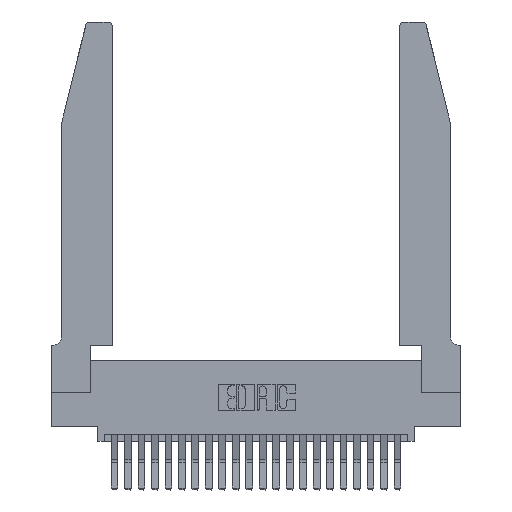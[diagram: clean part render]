
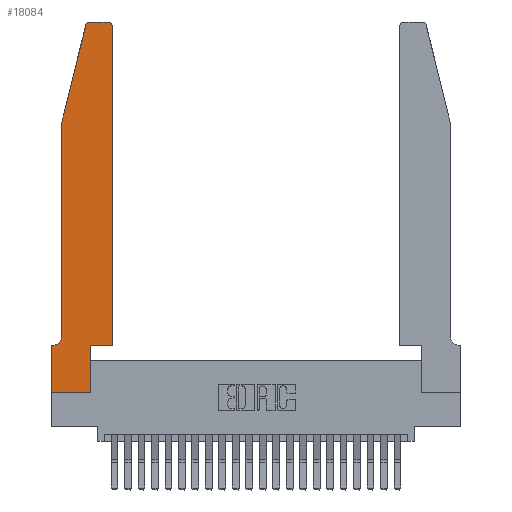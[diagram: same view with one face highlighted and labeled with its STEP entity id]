
A CAD part, top view. The second image highlights one B-rep face of the part: STEP entity #18084.
In plain terms, the highlighted planar face has unit normal (0, 0, 1).
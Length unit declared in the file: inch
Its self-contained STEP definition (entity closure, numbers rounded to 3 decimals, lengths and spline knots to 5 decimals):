
#71 = LINE ( 'NONE', #7031, #2191 ) ;
#272 = LINE ( 'NONE', #7744, #11992 ) ;
#812 = LINE ( 'NONE', #16373, #2931 ) ;
#839 = CARTESIAN_POINT ( 'NONE',  ( 0.0755, 0.42, 0.37 ) ) ;
#1042 = VERTEX_POINT ( 'NONE', #2028 ) ;
#1114 = EDGE_CURVE ( 'NONE', #1042, #7758, #5060, .T. ) ;
#1140 = LINE ( 'NONE', #19618, #18630 ) ;
#1260 = ORIENTED_EDGE ( 'NONE', *, *, #16427, .T. ) ;
#1825 = PLANE ( 'NONE',  #8593 ) ;
#2028 = CARTESIAN_POINT ( 'NONE',  ( 0.0755, 2., 0.37 ) ) ;
#2191 = VECTOR ( 'NONE', #20744, 39.37008 ) ;
#2342 = CARTESIAN_POINT ( 'NONE',  ( 0.25487, 2.72718, 0.37 ) ) ;
#2931 = VECTOR ( 'NONE', #18145, 39.37008 ) ;
#3253 = EDGE_CURVE ( 'NONE', #9945, #8658, #9412, .T. ) ;
#3567 = CARTESIAN_POINT ( 'NONE',  ( 0., 0.35, 0.37 ) ) ;
#3884 = CARTESIAN_POINT ( 'NONE',  ( 0.284, 2.72, 0.37 ) ) ;
#3889 = CARTESIAN_POINT ( 'NONE',  ( 0., 0.35, 0.37 ) ) ;
#4374 = LINE ( 'NONE', #8515, #10708 ) ;
#4862 = CARTESIAN_POINT ( 'NONE',  ( 0.4505, 2.72, 0.37 ) ) ;
#5060 = LINE ( 'NONE', #15901, #15611 ) ;
#5346 = ORIENTED_EDGE ( 'NONE', *, *, #16953, .T. ) ;
#5352 = CARTESIAN_POINT ( 'NONE',  ( 0.0755, 2., 0.37 ) ) ;
#5396 = VERTEX_POINT ( 'NONE', #23078 ) ;
#5805 = DIRECTION ( 'NONE',  ( 1., 0., 0. ) ) ;
#6069 = AXIS2_PLACEMENT_3D ( 'NONE', #3884, #11695, #5805 ) ;
#6329 = DIRECTION ( 'NONE',  ( 0., -1., 0. ) ) ;
#6452 = DIRECTION ( 'NONE',  ( 0., 0., 1. ) ) ;
#7031 = CARTESIAN_POINT ( 'NONE',  ( 0.0755, 0.35, 0.37 ) ) ;
#7457 = ORIENTED_EDGE ( 'NONE', *, *, #9416, .T. ) ;
#7469 = VERTEX_POINT ( 'NONE', #9758 ) ;
#7622 = VERTEX_POINT ( 'NONE', #24180 ) ;
#7744 = CARTESIAN_POINT ( 'NONE',  ( 0., 0., 0.37 ) ) ;
#7758 = VERTEX_POINT ( 'NONE', #839 ) ;
#7800 = CARTESIAN_POINT ( 'NONE',  ( 0.2865, 0.35, 0.37 ) ) ;
#7893 = DIRECTION ( 'NONE',  ( 1., 0., 0. ) ) ;
#8240 = EDGE_CURVE ( 'NONE', #11765, #8411, #20947, .T. ) ;
#8411 = VERTEX_POINT ( 'NONE', #24362 ) ;
#8515 = CARTESIAN_POINT ( 'NONE',  ( 0.4505, 0.35, 0.37 ) ) ;
#8593 = AXIS2_PLACEMENT_3D ( 'NONE', #3889, #19358, #7893 ) ;
#8658 = VERTEX_POINT ( 'NONE', #10297 ) ;
#9186 = DIRECTION ( 'NONE',  ( -0.239, -0.971, 0. ) ) ;
#9319 = VECTOR ( 'NONE', #9186, 39.37008 ) ;
#9412 = LINE ( 'NONE', #7800, #16129 ) ;
#9416 = EDGE_CURVE ( 'NONE', #15896, #7622, #9648, .T. ) ;
#9505 = ORIENTED_EDGE ( 'NONE', *, *, #12783, .T. ) ;
#9530 = CIRCLE ( 'NONE', #6069, 0.03 ) ;
#9648 = LINE ( 'NONE', #24105, #10263 ) ;
#9758 = CARTESIAN_POINT ( 'NONE',  ( 0.284, 2.75, 0.37 ) ) ;
#9945 = VERTEX_POINT ( 'NONE', #21659 ) ;
#10180 = EDGE_CURVE ( 'NONE', #12551, #1042, #14492, .T. ) ;
#10263 = VECTOR ( 'NONE', #14584, 39.37008 ) ;
#10297 = CARTESIAN_POINT ( 'NONE',  ( 0.2865, 0.35, 0.37 ) ) ;
#10518 = DIRECTION ( 'NONE',  ( -1., 0., 0. ) ) ;
#10708 = VECTOR ( 'NONE', #14386, 39.37008 ) ;
#10726 = AXIS2_PLACEMENT_3D ( 'NONE', #23954, #16304, #10518 ) ;
#11526 = DIRECTION ( 'NONE',  ( 0., 1., 0. ) ) ;
#11695 = DIRECTION ( 'NONE',  ( 0., 0., 1. ) ) ;
#11765 = VERTEX_POINT ( 'NONE', #4862 ) ;
#11797 = EDGE_LOOP ( 'NONE', ( #20360, #5346, #19533, #12193, #22420, #21292, #7457, #1260, #20268, #9505, #15422, #21900 ) ) ;
#11992 = VECTOR ( 'NONE', #17248, 39.37008 ) ;
#12193 = ORIENTED_EDGE ( 'NONE', *, *, #1114, .T. ) ;
#12444 = VERTEX_POINT ( 'NONE', #18569 ) ;
#12551 = VERTEX_POINT ( 'NONE', #2342 ) ;
#12661 = CARTESIAN_POINT ( 'NONE',  ( 0.4205, 2.72, 0.37 ) ) ;
#12783 = EDGE_CURVE ( 'NONE', #8658, #12444, #4374, .T. ) ;
#14386 = DIRECTION ( 'NONE',  ( 1., 0., 0. ) ) ;
#14475 = EDGE_CURVE ( 'NONE', #5396, #15896, #71, .T. ) ;
#14492 = LINE ( 'NONE', #5352, #9319 ) ;
#14551 = EDGE_CURVE ( 'NONE', #7758, #5396, #16968, .T. ) ;
#14584 = DIRECTION ( 'NONE',  ( 0., -1., 0. ) ) ;
#15422 = ORIENTED_EDGE ( 'NONE', *, *, #17434, .T. ) ;
#15611 = VECTOR ( 'NONE', #6329, 39.37008 ) ;
#15896 = VERTEX_POINT ( 'NONE', #3567 ) ;
#15901 = CARTESIAN_POINT ( 'NONE',  ( 0.0755, 2., 0.37 ) ) ;
#16129 = VECTOR ( 'NONE', #11526, 39.37008 ) ;
#16304 = DIRECTION ( 'NONE',  ( 0., 0., -1. ) ) ;
#16373 = CARTESIAN_POINT ( 'NONE',  ( 0.2605, 2.75, 0.37 ) ) ;
#16427 = EDGE_CURVE ( 'NONE', #7622, #9945, #272, .T. ) ;
#16953 = EDGE_CURVE ( 'NONE', #7469, #12551, #9530, .T. ) ;
#16968 = CIRCLE ( 'NONE', #10726, 0.07 ) ;
#17248 = DIRECTION ( 'NONE',  ( 1., 0., 0. ) ) ;
#17434 = EDGE_CURVE ( 'NONE', #12444, #11765, #1140, .T. ) ;
#18084 = ADVANCED_FACE ( 'NONE', ( #23686 ), #1825, .T. ) ;
#18145 = DIRECTION ( 'NONE',  ( -1., 0., 0. ) ) ;
#18324 = EDGE_CURVE ( 'NONE', #8411, #7469, #812, .T. ) ;
#18569 = CARTESIAN_POINT ( 'NONE',  ( 0.4505, 0.35, 0.37 ) ) ;
#18630 = VECTOR ( 'NONE', #19779, 39.37008 ) ;
#19358 = DIRECTION ( 'NONE',  ( 0., 0., 1. ) ) ;
#19533 = ORIENTED_EDGE ( 'NONE', *, *, #10180, .T. ) ;
#19618 = CARTESIAN_POINT ( 'NONE',  ( 0.4505, 0.35, 0.37 ) ) ;
#19779 = DIRECTION ( 'NONE',  ( 0., 1., 0. ) ) ;
#20268 = ORIENTED_EDGE ( 'NONE', *, *, #3253, .T. ) ;
#20360 = ORIENTED_EDGE ( 'NONE', *, *, #18324, .T. ) ;
#20744 = DIRECTION ( 'NONE',  ( -1., 0., 0. ) ) ;
#20947 = CIRCLE ( 'NONE', #22142, 0.03 ) ;
#21292 = ORIENTED_EDGE ( 'NONE', *, *, #14475, .T. ) ;
#21659 = CARTESIAN_POINT ( 'NONE',  ( 0.2865, 0., 0.37 ) ) ;
#21900 = ORIENTED_EDGE ( 'NONE', *, *, #8240, .T. ) ;
#22142 = AXIS2_PLACEMENT_3D ( 'NONE', #12661, #6452, #24046 ) ;
#22420 = ORIENTED_EDGE ( 'NONE', *, *, #14551, .T. ) ;
#23078 = CARTESIAN_POINT ( 'NONE',  ( 0.0055, 0.35, 0.37 ) ) ;
#23686 = FACE_OUTER_BOUND ( 'NONE', #11797, .T. ) ;
#23954 = CARTESIAN_POINT ( 'NONE',  ( 0.0055, 0.42, 0.37 ) ) ;
#24046 = DIRECTION ( 'NONE',  ( 1., 0., 0. ) ) ;
#24105 = CARTESIAN_POINT ( 'NONE',  ( 0., 0., 0.37 ) ) ;
#24180 = CARTESIAN_POINT ( 'NONE',  ( 0., 0., 0.37 ) ) ;
#24362 = CARTESIAN_POINT ( 'NONE',  ( 0.4205, 2.75, 0.37 ) ) ;
